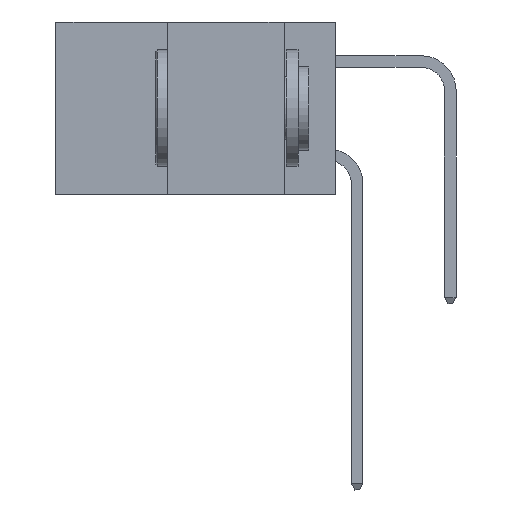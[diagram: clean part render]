
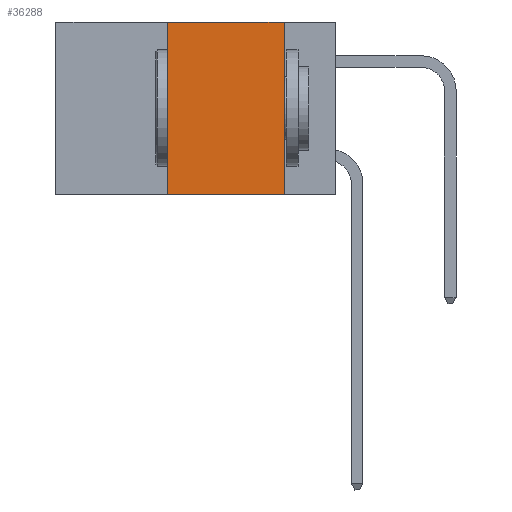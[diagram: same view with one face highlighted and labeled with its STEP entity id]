
A CAD part, left-side view. The second image highlights one B-rep face of the part: STEP entity #36288.
In plain terms, the highlighted planar face has unit normal (-1, 0, 0).
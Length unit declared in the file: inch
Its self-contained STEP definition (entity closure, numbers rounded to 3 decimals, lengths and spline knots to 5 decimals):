
#2155 = LINE ( 'NONE', #2684, #24910 ) ;
#2684 = CARTESIAN_POINT ( 'NONE',  ( 0., 0.36, 0. ) ) ;
#3406 = VERTEX_POINT ( 'NONE', #13776 ) ;
#4513 = PLANE ( 'NONE',  #10521 ) ;
#4574 = ORIENTED_EDGE ( 'NONE', *, *, #32784, .F. ) ;
#5191 = FACE_OUTER_BOUND ( 'NONE', #11859, .T. ) ;
#5555 = DIRECTION ( 'NONE',  ( 0., 0., 1. ) ) ;
#5819 = LINE ( 'NONE', #9071, #20097 ) ;
#5928 = VECTOR ( 'NONE', #7846, 39.37008 ) ;
#6345 = ORIENTED_EDGE ( 'NONE', *, *, #21799, .F. ) ;
#7296 = VERTEX_POINT ( 'NONE', #21770 ) ;
#7846 = DIRECTION ( 'NONE',  ( 0., -1., 0. ) ) ;
#9071 = CARTESIAN_POINT ( 'NONE',  ( 0., 0.11, 0. ) ) ;
#10521 = AXIS2_PLACEMENT_3D ( 'NONE', #13108, #32812, #15951 ) ;
#11859 = EDGE_LOOP ( 'NONE', ( #4574, #6345, #17500, #17964 ) ) ;
#13108 = CARTESIAN_POINT ( 'NONE',  ( 0., 0.6, 0. ) ) ;
#13776 = CARTESIAN_POINT ( 'NONE',  ( 0., 0.11, 0. ) ) ;
#13969 = VERTEX_POINT ( 'NONE', #15914 ) ;
#15914 = CARTESIAN_POINT ( 'NONE',  ( 0., 0.36, 0. ) ) ;
#15951 = DIRECTION ( 'NONE',  ( 0., 0., -1. ) ) ;
#17500 = ORIENTED_EDGE ( 'NONE', *, *, #25561, .F. ) ;
#17964 = ORIENTED_EDGE ( 'NONE', *, *, #22561, .T. ) ;
#18408 = CARTESIAN_POINT ( 'NONE',  ( 0., 0.36, -0.37 ) ) ;
#18571 = DIRECTION ( 'NONE',  ( 0., -1., 0. ) ) ;
#20097 = VECTOR ( 'NONE', #34470, 39.37008 ) ;
#21770 = CARTESIAN_POINT ( 'NONE',  ( 0., 0.11, -0.37 ) ) ;
#21799 = EDGE_CURVE ( 'NONE', #13969, #3406, #25201, .T. ) ;
#22011 = CARTESIAN_POINT ( 'NONE',  ( 0., 0.6, -0.37 ) ) ;
#22561 = EDGE_CURVE ( 'NONE', #34966, #7296, #34212, .T. ) ;
#24910 = VECTOR ( 'NONE', #5555, 39.37008 ) ;
#25201 = LINE ( 'NONE', #27106, #32574 ) ;
#25561 = EDGE_CURVE ( 'NONE', #34966, #13969, #2155, .T. ) ;
#27106 = CARTESIAN_POINT ( 'NONE',  ( 0., 0.6, 0. ) ) ;
#32574 = VECTOR ( 'NONE', #18571, 39.37008 ) ;
#32784 = EDGE_CURVE ( 'NONE', #3406, #7296, #5819, .T. ) ;
#32812 = DIRECTION ( 'NONE',  ( 1., 0., 0. ) ) ;
#34212 = LINE ( 'NONE', #22011, #5928 ) ;
#34470 = DIRECTION ( 'NONE',  ( 0., 0., -1. ) ) ;
#34966 = VERTEX_POINT ( 'NONE', #18408 ) ;
#36288 = ADVANCED_FACE ( 'NONE', ( #5191 ), #4513, .F. ) ;
